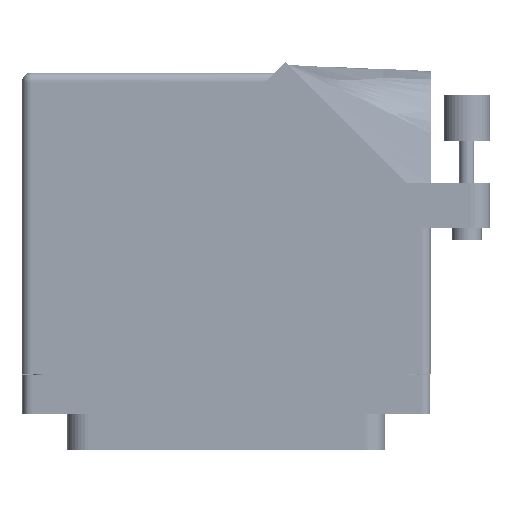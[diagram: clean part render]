
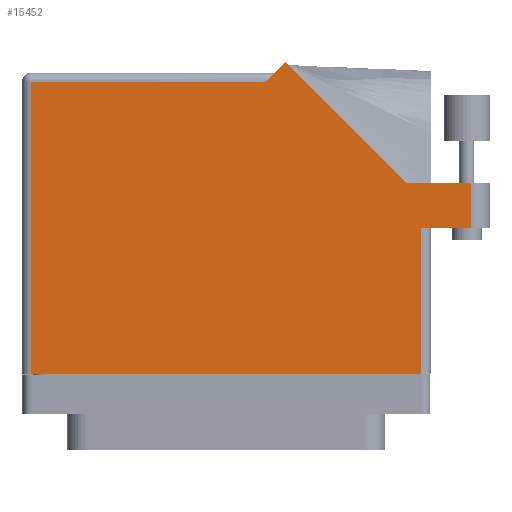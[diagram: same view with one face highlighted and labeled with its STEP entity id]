
A CAD part, front view. The second image highlights one B-rep face of the part: STEP entity #15452.
In plain terms, the highlighted face is planar.
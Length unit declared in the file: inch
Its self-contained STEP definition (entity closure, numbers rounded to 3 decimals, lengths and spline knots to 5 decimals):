
#602 = VECTOR ( 'NONE', #68996, 39.37008 ) ;
#2412 = PLANE ( 'NONE',  #11671 ) ;
#2940 = VECTOR ( 'NONE', #41449, 39.37008 ) ;
#3722 = CARTESIAN_POINT ( 'NONE',  ( -1.3155, 1.868, 0.765 ) ) ;
#5944 = VECTOR ( 'NONE', #62623, 39.37008 ) ;
#7858 = LINE ( 'NONE', #69648, #23611 ) ;
#9206 = EDGE_CURVE ( 'NONE', #22527, #21395, #22046, .T. ) ;
#10519 = CARTESIAN_POINT ( 'NONE',  ( 1.6525, 1.187, 0.765 ) ) ;
#11345 = CARTESIAN_POINT ( 'NONE',  ( 1.3155, -0.1, 0.765 ) ) ;
#11671 = AXIS2_PLACEMENT_3D ( 'NONE', #80792, #23155, #30647 ) ;
#13158 = CARTESIAN_POINT ( 'NONE',  ( 1.3155, 0.88, 0.765 ) ) ;
#14430 = ORIENTED_EDGE ( 'NONE', *, *, #35493, .T. ) ;
#14885 = VERTEX_POINT ( 'NONE', #36965 ) ;
#14941 = ORIENTED_EDGE ( 'NONE', *, *, #9206, .T. ) ;
#14977 = VERTEX_POINT ( 'NONE', #3722 ) ;
#15452 = ADVANCED_FACE ( 'NONE', ( #19241 ), #2412, .F. ) ;
#15676 = CARTESIAN_POINT ( 'NONE',  ( 0.39821, 2.00071, 0.765 ) ) ;
#15888 = ORIENTED_EDGE ( 'NONE', *, *, #65264, .T. ) ;
#19027 = ORIENTED_EDGE ( 'NONE', *, *, #83960, .T. ) ;
#19118 = ORIENTED_EDGE ( 'NONE', *, *, #54018, .T. ) ;
#19241 = FACE_OUTER_BOUND ( 'NONE', #55550, .T. ) ;
#20246 = CARTESIAN_POINT ( 'NONE',  ( -1.3775, 1.868, 0.765 ) ) ;
#21312 = DIRECTION ( 'NONE',  ( 0., 1., 0. ) ) ;
#21395 = VERTEX_POINT ( 'NONE', #90004 ) ;
#22046 = LINE ( 'NONE', #84437, #2940 ) ;
#22527 = VERTEX_POINT ( 'NONE', #15676 ) ;
#23155 = DIRECTION ( 'NONE',  ( 0., 0., -1. ) ) ;
#23611 = VECTOR ( 'NONE', #48278, 39.37008 ) ;
#30647 = DIRECTION ( 'NONE',  ( -1., 0., 0. ) ) ;
#30857 = DIRECTION ( 'NONE',  ( 1., 0., 0. ) ) ;
#32429 = EDGE_CURVE ( 'NONE', #14977, #48422, #61121, .T. ) ;
#33152 = LINE ( 'NONE', #82772, #602 ) ;
#35493 = EDGE_CURVE ( 'NONE', #48422, #88746, #49622, .T. ) ;
#36965 = CARTESIAN_POINT ( 'NONE',  ( 1.21192, 1.187, 0.765 ) ) ;
#38410 = EDGE_CURVE ( 'NONE', #14885, #22527, #50859, .T. ) ;
#41449 = DIRECTION ( 'NONE',  ( -0.707, -0.707, 0. ) ) ;
#45155 = CARTESIAN_POINT ( 'NONE',  ( 1.6525, 0.88, 0.765 ) ) ;
#48278 = DIRECTION ( 'NONE',  ( 1., 0., 0. ) ) ;
#48422 = VERTEX_POINT ( 'NONE', #55311 ) ;
#49622 = LINE ( 'NONE', #87927, #55211 ) ;
#50859 = LINE ( 'NONE', #84593, #5944 ) ;
#51715 = VERTEX_POINT ( 'NONE', #45155 ) ;
#52811 = VECTOR ( 'NONE', #61271, 39.37008 ) ;
#54018 = EDGE_CURVE ( 'NONE', #90882, #14885, #33152, .T. ) ;
#55211 = VECTOR ( 'NONE', #30857, 39.37008 ) ;
#55311 = CARTESIAN_POINT ( 'NONE',  ( -1.3155, -0.1, 0.765 ) ) ;
#55550 = EDGE_LOOP ( 'NONE', ( #77459, #19027, #19118, #68829, #14941, #81133, #73883, #14430, #15888 ) ) ;
#58394 = VECTOR ( 'NONE', #21312, 39.37008 ) ;
#58482 = CARTESIAN_POINT ( 'NONE',  ( -1.3155, -0.1, 0.765 ) ) ;
#61121 = LINE ( 'NONE', #58482, #90254 ) ;
#61271 = DIRECTION ( 'NONE',  ( 0., 1., 0. ) ) ;
#62623 = DIRECTION ( 'NONE',  ( -0.707, 0.707, 0. ) ) ;
#63618 = CARTESIAN_POINT ( 'NONE',  ( 1.3155, 0.88, 0.765 ) ) ;
#64957 = LINE ( 'NONE', #20246, #92898 ) ;
#65264 = EDGE_CURVE ( 'NONE', #88746, #65381, #87563, .T. ) ;
#65381 = VERTEX_POINT ( 'NONE', #13158 ) ;
#68032 = EDGE_CURVE ( 'NONE', #65381, #51715, #7858, .T. ) ;
#68829 = ORIENTED_EDGE ( 'NONE', *, *, #38410, .T. ) ;
#68996 = DIRECTION ( 'NONE',  ( -1., 0., 0. ) ) ;
#69648 = CARTESIAN_POINT ( 'NONE',  ( 1.3775, 0.88, 0.765 ) ) ;
#72925 = DIRECTION ( 'NONE',  ( 0., -1., 0. ) ) ;
#73056 = CARTESIAN_POINT ( 'NONE',  ( 1.6525, 1.187, 0.765 ) ) ;
#73883 = ORIENTED_EDGE ( 'NONE', *, *, #32429, .T. ) ;
#77459 = ORIENTED_EDGE ( 'NONE', *, *, #68032, .T. ) ;
#77617 = DIRECTION ( 'NONE',  ( -1., 0., 0. ) ) ;
#78311 = EDGE_CURVE ( 'NONE', #21395, #14977, #64957, .T. ) ;
#80792 = CARTESIAN_POINT ( 'NONE',  ( -1.3775, 1.93, 0.765 ) ) ;
#81133 = ORIENTED_EDGE ( 'NONE', *, *, #78311, .T. ) ;
#82772 = CARTESIAN_POINT ( 'NONE',  ( 1.7775, 1.187, 0.765 ) ) ;
#83167 = LINE ( 'NONE', #10519, #52811 ) ;
#83960 = EDGE_CURVE ( 'NONE', #51715, #90882, #83167, .T. ) ;
#84437 = CARTESIAN_POINT ( 'NONE',  ( 0.3275, 1.93, 0.765 ) ) ;
#84593 = CARTESIAN_POINT ( 'NONE',  ( 1.21192, 1.187, 0.765 ) ) ;
#87563 = LINE ( 'NONE', #63618, #58394 ) ;
#87927 = CARTESIAN_POINT ( 'NONE',  ( -1.3775, -0.1, 0.765 ) ) ;
#88746 = VERTEX_POINT ( 'NONE', #11345 ) ;
#90004 = CARTESIAN_POINT ( 'NONE',  ( 0.2655, 1.868, 0.765 ) ) ;
#90254 = VECTOR ( 'NONE', #72925, 39.37008 ) ;
#90882 = VERTEX_POINT ( 'NONE', #73056 ) ;
#92898 = VECTOR ( 'NONE', #77617, 39.37008 ) ;
